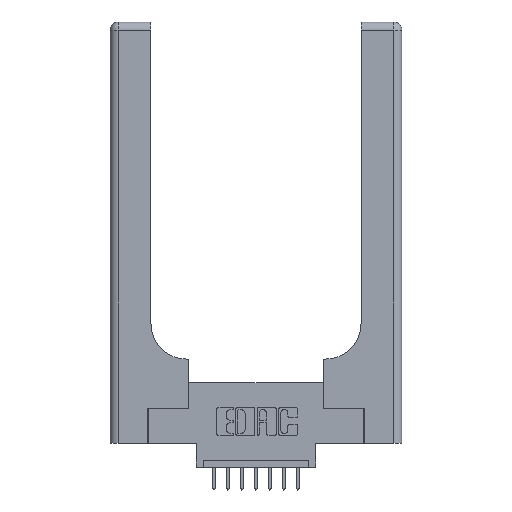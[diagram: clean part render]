
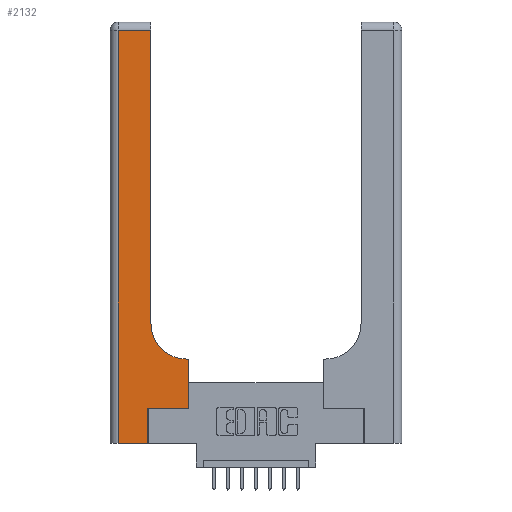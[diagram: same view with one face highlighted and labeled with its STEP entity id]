
A CAD part, top view. The second image highlights one B-rep face of the part: STEP entity #2132.
In plain terms, the highlighted planar face has unit normal (0, 0, 1).
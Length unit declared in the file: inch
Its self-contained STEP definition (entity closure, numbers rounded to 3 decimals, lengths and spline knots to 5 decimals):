
#74 = VECTOR ( 'NONE', #7682, 39.37008 ) ;
#168 = CARTESIAN_POINT ( 'NONE',  ( 0.2915, 0.6, 0.37 ) ) ;
#249 = DIRECTION ( 'NONE',  ( 0., 1., 0. ) ) ;
#293 = CARTESIAN_POINT ( 'NONE',  ( 0.269, 0., 0.37 ) ) ;
#506 = VECTOR ( 'NONE', #15161, 39.37008 ) ;
#934 = EDGE_CURVE ( 'NONE', #2828, #6031, #14551, .T. ) ;
#1033 = LINE ( 'NONE', #2705, #13808 ) ;
#1089 = EDGE_CURVE ( 'NONE', #6031, #3834, #10286, .T. ) ;
#1098 = ORIENTED_EDGE ( 'NONE', *, *, #3598, .T. ) ;
#1256 = DIRECTION ( 'NONE',  ( 0., 0., -1. ) ) ;
#1279 = CARTESIAN_POINT ( 'NONE',  ( 0.2915, 2.94, 0.37 ) ) ;
#1328 = DIRECTION ( 'NONE',  ( 1., 0., 0. ) ) ;
#1460 = DIRECTION ( 'NONE',  ( -1., 0., 0. ) ) ;
#2030 = ORIENTED_EDGE ( 'NONE', *, *, #934, .T. ) ;
#2132 = ADVANCED_FACE ( 'NONE', ( #3288 ), #7093, .F. ) ;
#2319 = CARTESIAN_POINT ( 'NONE',  ( 0.5585, 0.25, 0.37 ) ) ;
#2403 = CARTESIAN_POINT ( 'NONE',  ( 0.2915, 0.85, 0.37 ) ) ;
#2549 = VECTOR ( 'NONE', #1460, 39.37008 ) ;
#2705 = CARTESIAN_POINT ( 'NONE',  ( 0.5585, 0.25, 0.37 ) ) ;
#2730 = VERTEX_POINT ( 'NONE', #4929 ) ;
#2828 = VERTEX_POINT ( 'NONE', #293 ) ;
#2985 = CARTESIAN_POINT ( 'NONE',  ( 0.269, 0.25, 0.37 ) ) ;
#3094 = DIRECTION ( 'NONE',  ( 1., 0., 0. ) ) ;
#3240 = EDGE_CURVE ( 'NONE', #3834, #8832, #1033, .T. ) ;
#3269 = CARTESIAN_POINT ( 'NONE',  ( 0., 2.94, 0.37 ) ) ;
#3288 = FACE_OUTER_BOUND ( 'NONE', #7384, .T. ) ;
#3559 = VERTEX_POINT ( 'NONE', #1279 ) ;
#3598 = EDGE_CURVE ( 'NONE', #15200, #8730, #11945, .T. ) ;
#3834 = VERTEX_POINT ( 'NONE', #2319 ) ;
#4005 = ORIENTED_EDGE ( 'NONE', *, *, #5053, .T. ) ;
#4253 = CARTESIAN_POINT ( 'NONE',  ( 0.269, 0.25, 0.37 ) ) ;
#4327 = VECTOR ( 'NONE', #6741, 39.37008 ) ;
#4335 = LINE ( 'NONE', #11293, #74 ) ;
#4929 = CARTESIAN_POINT ( 'NONE',  ( 0.06, 0., 0.37 ) ) ;
#4936 = CARTESIAN_POINT ( 'NONE',  ( 0.5585, 0.6, 0.37 ) ) ;
#5047 = CARTESIAN_POINT ( 'NONE',  ( 0.269, 0., 0.37 ) ) ;
#5053 = EDGE_CURVE ( 'NONE', #9124, #2730, #10615, .T. ) ;
#5714 = LINE ( 'NONE', #168, #2549 ) ;
#6031 = VERTEX_POINT ( 'NONE', #4253 ) ;
#6062 = DIRECTION ( 'NONE',  ( -1., 0., 0. ) ) ;
#6269 = EDGE_CURVE ( 'NONE', #2730, #2828, #10747, .T. ) ;
#6308 = VECTOR ( 'NONE', #1328, 39.37008 ) ;
#6461 = ORIENTED_EDGE ( 'NONE', *, *, #12389, .T. ) ;
#6741 = DIRECTION ( 'NONE',  ( 0., -1., 0. ) ) ;
#7093 = PLANE ( 'NONE',  #8239 ) ;
#7384 = EDGE_LOOP ( 'NONE', ( #6461, #15197, #4005, #11317, #2030, #11120, #8622, #13170, #1098 ) ) ;
#7682 = DIRECTION ( 'NONE',  ( 0., 1., 0. ) ) ;
#7764 = CARTESIAN_POINT ( 'NONE',  ( 0., 0., 0.37 ) ) ;
#8112 = EDGE_CURVE ( 'NONE', #8832, #15200, #5714, .T. ) ;
#8239 = AXIS2_PLACEMENT_3D ( 'NONE', #14195, #1256, #6062 ) ;
#8622 = ORIENTED_EDGE ( 'NONE', *, *, #3240, .T. ) ;
#8730 = VERTEX_POINT ( 'NONE', #2403 ) ;
#8832 = VERTEX_POINT ( 'NONE', #4936 ) ;
#8835 = LINE ( 'NONE', #3269, #506 ) ;
#8998 = VECTOR ( 'NONE', #3094, 39.37008 ) ;
#9094 = CARTESIAN_POINT ( 'NONE',  ( 0.5415, 0.85, 0.37 ) ) ;
#9124 = VERTEX_POINT ( 'NONE', #10233 ) ;
#9955 = CARTESIAN_POINT ( 'NONE',  ( 0.06, 3., 0.37 ) ) ;
#10028 = DIRECTION ( 'NONE',  ( 0., 0., -1. ) ) ;
#10233 = CARTESIAN_POINT ( 'NONE',  ( 0.06, 2.94, 0.37 ) ) ;
#10286 = LINE ( 'NONE', #2985, #8998 ) ;
#10615 = LINE ( 'NONE', #9955, #4327 ) ;
#10747 = LINE ( 'NONE', #7764, #6308 ) ;
#10773 = EDGE_CURVE ( 'NONE', #3559, #9124, #8835, .T. ) ;
#10818 = AXIS2_PLACEMENT_3D ( 'NONE', #9094, #10028, #13593 ) ;
#11120 = ORIENTED_EDGE ( 'NONE', *, *, #1089, .T. ) ;
#11293 = CARTESIAN_POINT ( 'NONE',  ( 0.2915, 3., 0.37 ) ) ;
#11317 = ORIENTED_EDGE ( 'NONE', *, *, #6269, .T. ) ;
#11774 = VECTOR ( 'NONE', #13334, 39.37008 ) ;
#11945 = CIRCLE ( 'NONE', #10818, 0.25 ) ;
#12230 = CARTESIAN_POINT ( 'NONE',  ( 0.5415, 0.6, 0.37 ) ) ;
#12389 = EDGE_CURVE ( 'NONE', #8730, #3559, #4335, .T. ) ;
#13170 = ORIENTED_EDGE ( 'NONE', *, *, #8112, .T. ) ;
#13334 = DIRECTION ( 'NONE',  ( 0., 1., 0. ) ) ;
#13593 = DIRECTION ( 'NONE',  ( 1., 0., 0. ) ) ;
#13808 = VECTOR ( 'NONE', #249, 39.37008 ) ;
#14195 = CARTESIAN_POINT ( 'NONE',  ( 0., 3., 0.37 ) ) ;
#14551 = LINE ( 'NONE', #5047, #11774 ) ;
#15161 = DIRECTION ( 'NONE',  ( -1., 0., 0. ) ) ;
#15197 = ORIENTED_EDGE ( 'NONE', *, *, #10773, .T. ) ;
#15200 = VERTEX_POINT ( 'NONE', #12230 ) ;
